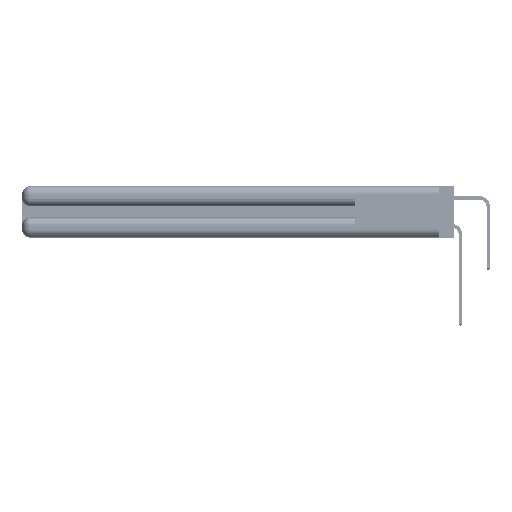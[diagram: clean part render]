
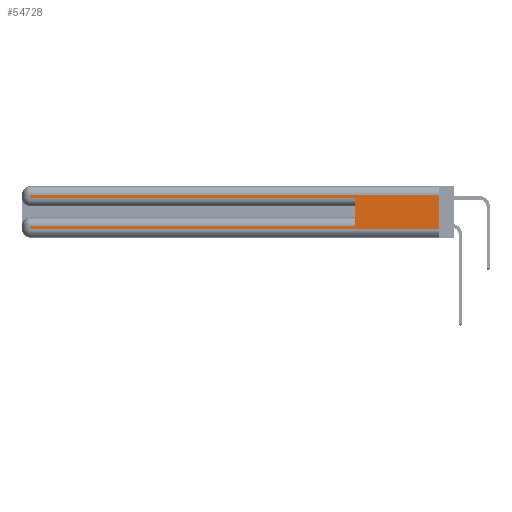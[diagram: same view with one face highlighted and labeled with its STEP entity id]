
A CAD part, left-side view. The second image highlights one B-rep face of the part: STEP entity #54728.
In plain terms, the highlighted planar face has unit normal (-1, 0, 0).
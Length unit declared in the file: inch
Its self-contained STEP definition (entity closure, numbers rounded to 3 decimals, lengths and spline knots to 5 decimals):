
#409 = EDGE_LOOP ( 'NONE', ( #28102, #9350, #47588, #7217, #21732, #17551, #37717, #32105 ) ) ;
#1118 = EDGE_CURVE ( 'NONE', #30620, #9208, #2209, .T. ) ;
#1320 = DIRECTION ( 'NONE',  ( 0., 0., 1. ) ) ;
#2209 = LINE ( 'NONE', #51558, #54303 ) ;
#2840 = VERTEX_POINT ( 'NONE', #27679 ) ;
#3318 = EDGE_CURVE ( 'NONE', #48470, #2840, #42032, .T. ) ;
#4340 = CARTESIAN_POINT ( 'NONE',  ( 0., 2.94, 0.085 ) ) ;
#5395 = CARTESIAN_POINT ( 'NONE',  ( 0., 0.6, 0.285 ) ) ;
#6447 = CARTESIAN_POINT ( 'NONE',  ( 0., 2.94, 0.285 ) ) ;
#6474 = LINE ( 'NONE', #12841, #19662 ) ;
#6574 = VECTOR ( 'NONE', #52667, 39.37008 ) ;
#7217 = ORIENTED_EDGE ( 'NONE', *, *, #1118, .T. ) ;
#8065 = LINE ( 'NONE', #37582, #18455 ) ;
#8275 = LINE ( 'NONE', #50487, #9651 ) ;
#9208 = VERTEX_POINT ( 'NONE', #5395 ) ;
#9350 = ORIENTED_EDGE ( 'NONE', *, *, #45783, .T. ) ;
#9651 = VECTOR ( 'NONE', #37111, 39.37008 ) ;
#10516 = VECTOR ( 'NONE', #55205, 39.37008 ) ;
#12841 = CARTESIAN_POINT ( 'NONE',  ( 0., 0., 0.31 ) ) ;
#17077 = EDGE_CURVE ( 'NONE', #37245, #9208, #21687, .T. ) ;
#17551 = ORIENTED_EDGE ( 'NONE', *, *, #50966, .T. ) ;
#17722 = CARTESIAN_POINT ( 'NONE',  ( 0., 2.94, 0.31 ) ) ;
#18455 = VECTOR ( 'NONE', #46718, 39.37008 ) ;
#18963 = EDGE_CURVE ( 'NONE', #20012, #30620, #8275, .T. ) ;
#19662 = VECTOR ( 'NONE', #43932, 39.37008 ) ;
#20012 = VERTEX_POINT ( 'NONE', #17722 ) ;
#21687 = LINE ( 'NONE', #54516, #55729 ) ;
#21732 = ORIENTED_EDGE ( 'NONE', *, *, #17077, .F. ) ;
#22670 = VERTEX_POINT ( 'NONE', #4340 ) ;
#23810 = EDGE_CURVE ( 'NONE', #56118, #2840, #38372, .T. ) ;
#25340 = DIRECTION ( 'NONE',  ( 0., 0., -1. ) ) ;
#25874 = CARTESIAN_POINT ( 'NONE',  ( 0., 0., 0.06 ) ) ;
#26503 = VECTOR ( 'NONE', #40322, 39.37008 ) ;
#27679 = CARTESIAN_POINT ( 'NONE',  ( 0., 0., 0.06 ) ) ;
#28102 = ORIENTED_EDGE ( 'NONE', *, *, #23810, .F. ) ;
#30101 = EDGE_CURVE ( 'NONE', #22670, #48470, #8065, .T. ) ;
#30620 = VERTEX_POINT ( 'NONE', #6447 ) ;
#32105 = ORIENTED_EDGE ( 'NONE', *, *, #3318, .T. ) ;
#34093 = CARTESIAN_POINT ( 'NONE',  ( 0., 0., 0.37 ) ) ;
#36062 = CARTESIAN_POINT ( 'NONE',  ( 0., 0., 0.31 ) ) ;
#36117 = AXIS2_PLACEMENT_3D ( 'NONE', #34093, #51942, #25340 ) ;
#37111 = DIRECTION ( 'NONE',  ( 0., 0., -1. ) ) ;
#37245 = VERTEX_POINT ( 'NONE', #54067 ) ;
#37582 = CARTESIAN_POINT ( 'NONE',  ( 0., 2.94, 0.37 ) ) ;
#37717 = ORIENTED_EDGE ( 'NONE', *, *, #30101, .T. ) ;
#38372 = LINE ( 'NONE', #53509, #26503 ) ;
#40322 = DIRECTION ( 'NONE',  ( 0., 0., -1. ) ) ;
#42032 = LINE ( 'NONE', #25874, #6574 ) ;
#43006 = FACE_OUTER_BOUND ( 'NONE', #409, .T. ) ;
#43932 = DIRECTION ( 'NONE',  ( 0., 1., 0. ) ) ;
#45783 = EDGE_CURVE ( 'NONE', #56118, #20012, #6474, .T. ) ;
#45990 = LINE ( 'NONE', #50778, #10516 ) ;
#46718 = DIRECTION ( 'NONE',  ( 0., 0., -1. ) ) ;
#47525 = PLANE ( 'NONE',  #36117 ) ;
#47588 = ORIENTED_EDGE ( 'NONE', *, *, #18963, .T. ) ;
#48470 = VERTEX_POINT ( 'NONE', #54870 ) ;
#50487 = CARTESIAN_POINT ( 'NONE',  ( 0., 2.94, 0.37 ) ) ;
#50778 = CARTESIAN_POINT ( 'NONE',  ( 0., 0., 0.085 ) ) ;
#50966 = EDGE_CURVE ( 'NONE', #37245, #22670, #45990, .T. ) ;
#51558 = CARTESIAN_POINT ( 'NONE',  ( 0., 0., 0.285 ) ) ;
#51942 = DIRECTION ( 'NONE',  ( 1., 0., 0. ) ) ;
#52667 = DIRECTION ( 'NONE',  ( 0., -1., 0. ) ) ;
#53509 = CARTESIAN_POINT ( 'NONE',  ( 0., 0., 0.37 ) ) ;
#54067 = CARTESIAN_POINT ( 'NONE',  ( 0., 0.6, 0.085 ) ) ;
#54303 = VECTOR ( 'NONE', #55986, 39.37008 ) ;
#54516 = CARTESIAN_POINT ( 'NONE',  ( 0., 0.6, 0.145 ) ) ;
#54728 = ADVANCED_FACE ( 'NONE', ( #43006 ), #47525, .F. ) ;
#54870 = CARTESIAN_POINT ( 'NONE',  ( 0., 2.94, 0.06 ) ) ;
#55205 = DIRECTION ( 'NONE',  ( 0., 1., 0. ) ) ;
#55729 = VECTOR ( 'NONE', #1320, 39.37008 ) ;
#55986 = DIRECTION ( 'NONE',  ( 0., -1., 0. ) ) ;
#56118 = VERTEX_POINT ( 'NONE', #36062 ) ;
